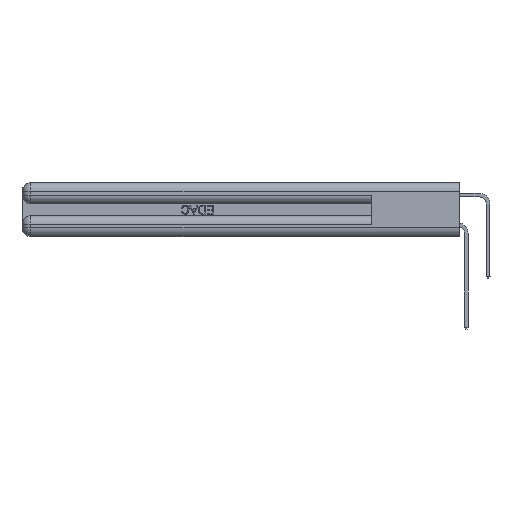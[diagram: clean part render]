
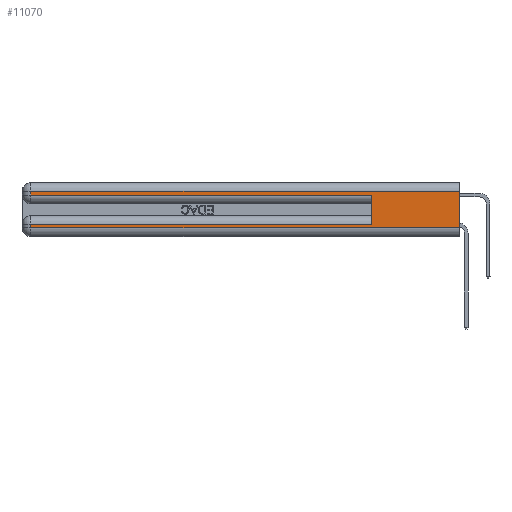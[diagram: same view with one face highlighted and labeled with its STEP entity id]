
A CAD part, left-side view. The second image highlights one B-rep face of the part: STEP entity #11070.
In plain terms, the highlighted planar face has unit normal (-1, 0, 0).
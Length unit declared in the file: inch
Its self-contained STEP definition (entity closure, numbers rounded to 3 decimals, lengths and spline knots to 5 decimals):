
#313 = EDGE_CURVE ( 'NONE', #33110, #1384, #12952, .T. ) ;
#619 = EDGE_CURVE ( 'NONE', #42915, #1384, #3258, .T. ) ;
#949 = ORIENTED_EDGE ( 'NONE', *, *, #28997, .T. ) ;
#1384 = VERTEX_POINT ( 'NONE', #33267 ) ;
#1643 = DIRECTION ( 'NONE',  ( 0., 0., -1. ) ) ;
#2463 = CARTESIAN_POINT ( 'NONE',  ( 0., 2.94, 0.37 ) ) ;
#2663 = ORIENTED_EDGE ( 'NONE', *, *, #26722, .T. ) ;
#3258 = LINE ( 'NONE', #31499, #3758 ) ;
#3337 = CARTESIAN_POINT ( 'NONE',  ( 0., 0., 0.285 ) ) ;
#3758 = VECTOR ( 'NONE', #34749, 39.37008 ) ;
#4191 = EDGE_LOOP ( 'NONE', ( #14599, #949, #7204, #36833, #31470, #41602, #21852, #2663 ) ) ;
#4267 = DIRECTION ( 'NONE',  ( 0., 0., -1. ) ) ;
#5797 = VECTOR ( 'NONE', #25583, 39.37008 ) ;
#5857 = VERTEX_POINT ( 'NONE', #43044 ) ;
#6093 = VECTOR ( 'NONE', #1643, 39.37008 ) ;
#6243 = FACE_OUTER_BOUND ( 'NONE', #4191, .T. ) ;
#7204 = ORIENTED_EDGE ( 'NONE', *, *, #11981, .T. ) ;
#7332 = PLANE ( 'NONE',  #23708 ) ;
#7770 = LINE ( 'NONE', #39822, #25512 ) ;
#8668 = DIRECTION ( 'NONE',  ( 0., -1., 0. ) ) ;
#10401 = EDGE_CURVE ( 'NONE', #36168, #10405, #14359, .T. ) ;
#10405 = VERTEX_POINT ( 'NONE', #41575 ) ;
#11070 = ADVANCED_FACE ( 'NONE', ( #6243 ), #7332, .F. ) ;
#11495 = CARTESIAN_POINT ( 'NONE',  ( 0., 2.94, 0.37 ) ) ;
#11531 = VECTOR ( 'NONE', #22433, 39.37008 ) ;
#11738 = CARTESIAN_POINT ( 'NONE',  ( 0., 0.6, 0.085 ) ) ;
#11981 = EDGE_CURVE ( 'NONE', #16679, #33110, #36139, .T. ) ;
#12952 = LINE ( 'NONE', #3337, #17706 ) ;
#13010 = CARTESIAN_POINT ( 'NONE',  ( 0., 2.94, 0.285 ) ) ;
#13321 = LINE ( 'NONE', #32036, #30005 ) ;
#14359 = LINE ( 'NONE', #11495, #31039 ) ;
#14599 = ORIENTED_EDGE ( 'NONE', *, *, #16125, .F. ) ;
#14738 = CARTESIAN_POINT ( 'NONE',  ( 0., 2.94, 0.085 ) ) ;
#14889 = LINE ( 'NONE', #32145, #5797 ) ;
#15177 = VERTEX_POINT ( 'NONE', #17149 ) ;
#16125 = EDGE_CURVE ( 'NONE', #5857, #15177, #21632, .T. ) ;
#16679 = VERTEX_POINT ( 'NONE', #17406 ) ;
#17149 = CARTESIAN_POINT ( 'NONE',  ( 0., 0., 0.06 ) ) ;
#17406 = CARTESIAN_POINT ( 'NONE',  ( 0., 2.94, 0.31 ) ) ;
#17706 = VECTOR ( 'NONE', #18219, 39.37008 ) ;
#18219 = DIRECTION ( 'NONE',  ( 0., -1., 0. ) ) ;
#19282 = DIRECTION ( 'NONE',  ( 1., 0., 0. ) ) ;
#21549 = DIRECTION ( 'NONE',  ( 0., 0., -1. ) ) ;
#21632 = LINE ( 'NONE', #22192, #6093 ) ;
#21852 = ORIENTED_EDGE ( 'NONE', *, *, #10401, .T. ) ;
#22192 = CARTESIAN_POINT ( 'NONE',  ( 0., 0., 0.37 ) ) ;
#22433 = DIRECTION ( 'NONE',  ( 0., 0., -1. ) ) ;
#22805 = DIRECTION ( 'NONE',  ( 0., 1., 0. ) ) ;
#23068 = EDGE_CURVE ( 'NONE', #42915, #36168, #7770, .T. ) ;
#23708 = AXIS2_PLACEMENT_3D ( 'NONE', #24704, #19282, #4267 ) ;
#24704 = CARTESIAN_POINT ( 'NONE',  ( 0., 0., 0.37 ) ) ;
#25512 = VECTOR ( 'NONE', #22805, 39.37008 ) ;
#25583 = DIRECTION ( 'NONE',  ( 0., 1., 0. ) ) ;
#26722 = EDGE_CURVE ( 'NONE', #10405, #15177, #13321, .T. ) ;
#28997 = EDGE_CURVE ( 'NONE', #5857, #16679, #14889, .T. ) ;
#30005 = VECTOR ( 'NONE', #8668, 39.37008 ) ;
#31039 = VECTOR ( 'NONE', #21549, 39.37008 ) ;
#31470 = ORIENTED_EDGE ( 'NONE', *, *, #619, .F. ) ;
#31499 = CARTESIAN_POINT ( 'NONE',  ( 0., 0.6, 0.145 ) ) ;
#32036 = CARTESIAN_POINT ( 'NONE',  ( 0., 0., 0.06 ) ) ;
#32145 = CARTESIAN_POINT ( 'NONE',  ( 0., 0., 0.31 ) ) ;
#33110 = VERTEX_POINT ( 'NONE', #13010 ) ;
#33267 = CARTESIAN_POINT ( 'NONE',  ( 0., 0.6, 0.285 ) ) ;
#34749 = DIRECTION ( 'NONE',  ( 0., 0., 1. ) ) ;
#36139 = LINE ( 'NONE', #2463, #11531 ) ;
#36168 = VERTEX_POINT ( 'NONE', #14738 ) ;
#36833 = ORIENTED_EDGE ( 'NONE', *, *, #313, .T. ) ;
#39822 = CARTESIAN_POINT ( 'NONE',  ( 0., 0., 0.085 ) ) ;
#41575 = CARTESIAN_POINT ( 'NONE',  ( 0., 2.94, 0.06 ) ) ;
#41602 = ORIENTED_EDGE ( 'NONE', *, *, #23068, .T. ) ;
#42915 = VERTEX_POINT ( 'NONE', #11738 ) ;
#43044 = CARTESIAN_POINT ( 'NONE',  ( 0., 0., 0.31 ) ) ;
